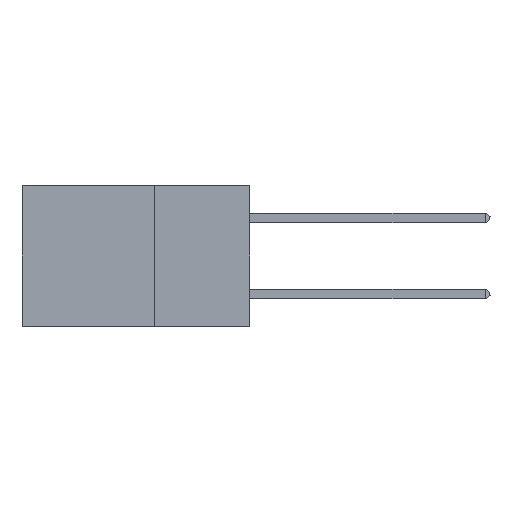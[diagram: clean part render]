
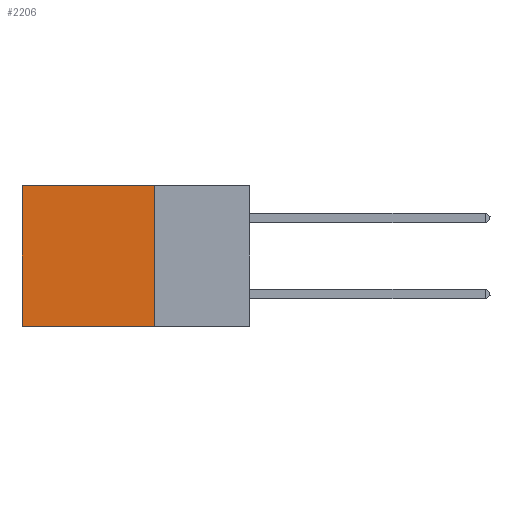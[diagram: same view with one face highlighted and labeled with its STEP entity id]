
A CAD part, left-side view. The second image highlights one B-rep face of the part: STEP entity #2206.
In plain terms, the highlighted planar face has unit normal (-1, 0, 0).
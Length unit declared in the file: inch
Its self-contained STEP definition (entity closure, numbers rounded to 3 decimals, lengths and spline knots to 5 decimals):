
#1847 = DIRECTION ( 'NONE',  ( 1., 0., 0. ) ) ;
#2206 = ADVANCED_FACE ( 'NONE', ( #14005 ), #4764, .F. ) ;
#2237 = DIRECTION ( 'NONE',  ( 0., 0., -1. ) ) ;
#2912 = EDGE_CURVE ( 'NONE', #43283, #14857, #10026, .T. ) ;
#4764 = PLANE ( 'NONE',  #25113 ) ;
#5475 = CARTESIAN_POINT ( 'NONE',  ( 0.2875, 0.25, 0. ) ) ;
#9683 = EDGE_CURVE ( 'NONE', #43283, #36054, #15484, .T. ) ;
#10026 = LINE ( 'NONE', #5475, #27533 ) ;
#10975 = ORIENTED_EDGE ( 'NONE', *, *, #15331, .T. ) ;
#11742 = VERTEX_POINT ( 'NONE', #15711 ) ;
#11766 = ORIENTED_EDGE ( 'NONE', *, *, #25188, .F. ) ;
#12073 = DIRECTION ( 'NONE',  ( 0., 0., -1. ) ) ;
#12615 = CARTESIAN_POINT ( 'NONE',  ( 0.2875, 0.6, 0. ) ) ;
#13414 = CARTESIAN_POINT ( 'NONE',  ( 0.2875, 0.6, 0. ) ) ;
#13951 = VECTOR ( 'NONE', #20031, 39.37008 ) ;
#14005 = FACE_OUTER_BOUND ( 'NONE', #35869, .T. ) ;
#14857 = VERTEX_POINT ( 'NONE', #13414 ) ;
#15331 = EDGE_CURVE ( 'NONE', #14857, #11742, #18147, .T. ) ;
#15409 = CARTESIAN_POINT ( 'NONE',  ( 0.2875, 0.25, -0.37 ) ) ;
#15484 = LINE ( 'NONE', #30120, #37964 ) ;
#15711 = CARTESIAN_POINT ( 'NONE',  ( 0.2875, 0.6, -0.37 ) ) ;
#18147 = LINE ( 'NONE', #12615, #24158 ) ;
#20031 = DIRECTION ( 'NONE',  ( 0., 1., 0. ) ) ;
#22746 = CARTESIAN_POINT ( 'NONE',  ( 0.2875, 0.25, 0. ) ) ;
#23757 = CARTESIAN_POINT ( 'NONE',  ( 0.2875, 0.25, 0. ) ) ;
#24158 = VECTOR ( 'NONE', #2237, 39.37008 ) ;
#25113 = AXIS2_PLACEMENT_3D ( 'NONE', #22746, #1847, #12073 ) ;
#25188 = EDGE_CURVE ( 'NONE', #36054, #11742, #42483, .T. ) ;
#27533 = VECTOR ( 'NONE', #40407, 39.37008 ) ;
#30120 = CARTESIAN_POINT ( 'NONE',  ( 0.2875, 0.25, 0. ) ) ;
#33793 = DIRECTION ( 'NONE',  ( 0., 0., -1. ) ) ;
#35127 = ORIENTED_EDGE ( 'NONE', *, *, #2912, .T. ) ;
#35869 = EDGE_LOOP ( 'NONE', ( #10975, #11766, #36743, #35127 ) ) ;
#36054 = VERTEX_POINT ( 'NONE', #15409 ) ;
#36743 = ORIENTED_EDGE ( 'NONE', *, *, #9683, .F. ) ;
#37964 = VECTOR ( 'NONE', #33793, 39.37008 ) ;
#40407 = DIRECTION ( 'NONE',  ( 0., 1., 0. ) ) ;
#41092 = CARTESIAN_POINT ( 'NONE',  ( 0.2875, 0.25, -0.37 ) ) ;
#42483 = LINE ( 'NONE', #41092, #13951 ) ;
#43283 = VERTEX_POINT ( 'NONE', #23757 ) ;
